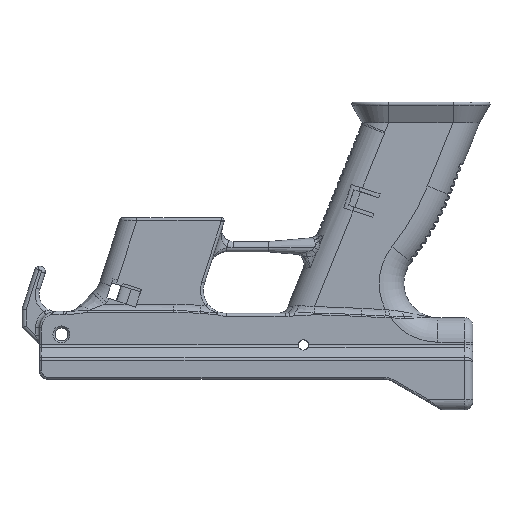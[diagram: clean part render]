
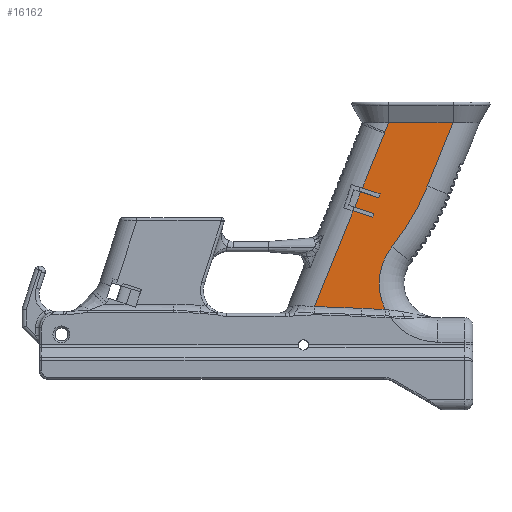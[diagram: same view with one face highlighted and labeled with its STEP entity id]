
A CAD part, front view. The second image highlights one B-rep face of the part: STEP entity #16162.
In plain terms, the highlighted planar face has unit normal (0, -1, 0).
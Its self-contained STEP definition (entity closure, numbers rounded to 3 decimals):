
#1591=FACE_OUTER_BOUND('',#2567,.T.);
#2567=EDGE_LOOP('',(#12655,#12656,#12657,#12658,#12659,#12660,#12661,#12662,
#12663,#12664,#12665,#12666,#12667,#12668,#12669,#12670,#12671));
#3439=CIRCLE('',#17698,696.304);
#3440=CIRCLE('',#17699,689.416);
#3441=CIRCLE('',#17700,28.63);
#3442=CIRCLE('',#17701,118.894);
#3443=CIRCLE('',#17702,17.);
#4932=LINE('',#29769,#5874);
#4947=LINE('',#29909,#5889);
#4948=LINE('',#29917,#5890);
#4990=LINE('',#31577,#5932);
#4991=LINE('',#31579,#5933);
#4992=LINE('',#31580,#5934);
#4993=LINE('',#31589,#5935);
#4994=LINE('',#31591,#5936);
#4995=LINE('',#31594,#5937);
#4996=LINE('',#31596,#5938);
#4997=LINE('',#31598,#5939);
#4998=LINE('',#31599,#5940);
#5874=VECTOR('',#20651,1000.);
#5889=VECTOR('',#20726,1000.);
#5890=VECTOR('',#20733,1000.);
#5932=VECTOR('',#20863,1000.);
#5933=VECTOR('',#20864,1000.);
#5934=VECTOR('',#20865,1000.);
#5935=VECTOR('',#20874,1000.);
#5936=VECTOR('',#20875,1000.);
#5937=VECTOR('',#20878,1000.);
#5938=VECTOR('',#20879,1000.);
#5939=VECTOR('',#20880,1000.);
#5940=VECTOR('',#20881,1000.);
#7390=VERTEX_POINT('',#29734);
#7392=VERTEX_POINT('',#29768);
#7418=VERTEX_POINT('',#29901);
#7419=VERTEX_POINT('',#29908);
#7422=VERTEX_POINT('',#29914);
#7423=VERTEX_POINT('',#29916);
#7505=VERTEX_POINT('',#31575);
#7506=VERTEX_POINT('',#31576);
#7507=VERTEX_POINT('',#31578);
#7508=VERTEX_POINT('',#31581);
#7509=VERTEX_POINT('',#31583);
#7510=VERTEX_POINT('',#31585);
#7511=VERTEX_POINT('',#31588);
#7512=VERTEX_POINT('',#31590);
#7513=VERTEX_POINT('',#31593);
#7514=VERTEX_POINT('',#31595);
#7515=VERTEX_POINT('',#31597);
#9336=EDGE_CURVE('',#7390,#7392,#4932,.T.);
#9378=EDGE_CURVE('',#7418,#7419,#4947,.T.);
#9382=EDGE_CURVE('',#7422,#7423,#4948,.T.);
#9511=EDGE_CURVE('',#7505,#7506,#4990,.T.);
#9512=EDGE_CURVE('',#7505,#7507,#4991,.T.);
#9513=EDGE_CURVE('',#7507,#7419,#4992,.T.);
#9514=EDGE_CURVE('',#7508,#7418,#3439,.T.);
#9515=EDGE_CURVE('',#7509,#7508,#3440,.T.);
#9516=EDGE_CURVE('',#7510,#7509,#3441,.T.);
#9517=EDGE_CURVE('',#7392,#7510,#3442,.T.);
#9518=EDGE_CURVE('',#7511,#7390,#4993,.T.);
#9519=EDGE_CURVE('',#7511,#7512,#4994,.T.);
#9520=EDGE_CURVE('',#7423,#7512,#3443,.T.);
#9521=EDGE_CURVE('',#7422,#7513,#4995,.T.);
#9522=EDGE_CURVE('',#7513,#7514,#4996,.T.);
#9523=EDGE_CURVE('',#7515,#7514,#4997,.T.);
#9524=EDGE_CURVE('',#7506,#7515,#4998,.T.);
#12655=ORIENTED_EDGE('',*,*,#9511,.F.);
#12656=ORIENTED_EDGE('',*,*,#9512,.T.);
#12657=ORIENTED_EDGE('',*,*,#9513,.T.);
#12658=ORIENTED_EDGE('',*,*,#9378,.F.);
#12659=ORIENTED_EDGE('',*,*,#9514,.F.);
#12660=ORIENTED_EDGE('',*,*,#9515,.F.);
#12661=ORIENTED_EDGE('',*,*,#9516,.F.);
#12662=ORIENTED_EDGE('',*,*,#9517,.F.);
#12663=ORIENTED_EDGE('',*,*,#9336,.F.);
#12664=ORIENTED_EDGE('',*,*,#9518,.F.);
#12665=ORIENTED_EDGE('',*,*,#9519,.T.);
#12666=ORIENTED_EDGE('',*,*,#9520,.F.);
#12667=ORIENTED_EDGE('',*,*,#9382,.F.);
#12668=ORIENTED_EDGE('',*,*,#9521,.T.);
#12669=ORIENTED_EDGE('',*,*,#9522,.T.);
#12670=ORIENTED_EDGE('',*,*,#9523,.F.);
#12671=ORIENTED_EDGE('',*,*,#9524,.F.);
#15610=PLANE('',#17697);
#16162=ADVANCED_FACE('',(#1591),#15610,.T.);
#17697=AXIS2_PLACEMENT_3D('',#31574,#20861,#20862);
#17698=AXIS2_PLACEMENT_3D('',#31582,#20866,#20867);
#17699=AXIS2_PLACEMENT_3D('',#31584,#20868,#20869);
#17700=AXIS2_PLACEMENT_3D('',#31586,#20870,#20871);
#17701=AXIS2_PLACEMENT_3D('',#31587,#20872,#20873);
#17702=AXIS2_PLACEMENT_3D('',#31592,#20876,#20877);
#20651=DIRECTION('',(-0.375,0.,-0.927));
#20726=DIRECTION('',(0.375,0.,0.927));
#20733=DIRECTION('',(0.375,0.,0.927));
#20861=DIRECTION('center_axis',(0.,-1.,0.));
#20862=DIRECTION('ref_axis',(0.,0.,-1.));
#20863=DIRECTION('',(-0.952,0.,0.305));
#20864=DIRECTION('',(-0.305,0.,-0.952));
#20865=DIRECTION('',(-0.952,0.,0.305));
#20866=DIRECTION('center_axis',(0.,-1.,0.));
#20867=DIRECTION('ref_axis',(-0.054,0.,-0.999));
#20868=DIRECTION('center_axis',(0.,1.,0.));
#20869=DIRECTION('ref_axis',(0.037,0.,0.999));
#20870=DIRECTION('center_axis',(0.,-1.,0.));
#20871=DIRECTION('ref_axis',(0.782,0.,-0.624));
#20872=DIRECTION('center_axis',(0.,1.,0.));
#20873=DIRECTION('ref_axis',(0.891,0.,-0.454));
#20874=DIRECTION('',(1.,0.,0.));
#20875=DIRECTION('',(-0.375,0.,-0.927));
#20876=DIRECTION('center_axis',(0.,-1.,0.));
#20877=DIRECTION('ref_axis',(0.992,0.,0.126));
#20878=DIRECTION('',(0.952,0.,-0.305));
#20879=DIRECTION('',(-0.305,0.,-0.952));
#20880=DIRECTION('',(0.952,0.,-0.305));
#20881=DIRECTION('',(0.375,0.,0.927));
#29734=CARTESIAN_POINT('',(121.365,-14.625,27.958));
#29768=CARTESIAN_POINT('',(108.893,-14.625,-2.912));
#29769=CARTESIAN_POINT('',(111.761,-14.625,4.188));
#29901=CARTESIAN_POINT('',(53.832,-14.625,-61.703));
#29908=CARTESIAN_POINT('',(72.662,-14.625,-15.097));
#29909=CARTESIAN_POINT('',(70.22,-14.625,-21.141));
#29914=CARTESIAN_POINT('',(77.169,-14.625,-3.94));
#29916=CARTESIAN_POINT('',(87.937,-14.625,22.71));
#29917=CARTESIAN_POINT('',(70.22,-14.625,-21.141));
#31574=CARTESIAN_POINT('Origin',(86.464,-14.625,-15.081));
#31575=CARTESIAN_POINT('',(82.782,-14.625,-16.238));
#31576=CARTESIAN_POINT('',(73.413,-14.625,-13.237));
#31577=CARTESIAN_POINT('',(2.985,-14.625,9.32));
#31578=CARTESIAN_POINT('',(82.172,-14.625,-18.143));
#31579=CARTESIAN_POINT('',(79.797,-14.625,-25.559));
#31580=CARTESIAN_POINT('',(2.375,-14.625,7.416));
#31581=CARTESIAN_POINT('',(76.954,-14.625,-62.561));
#31582=CARTESIAN_POINT('Origin',(39.557,-14.625,-757.86));
#31583=CARTESIAN_POINT('',(88.326,-14.625,-63.079));
#31584=CARTESIAN_POINT('Origin',(113.981,-14.625,625.86));
#31585=CARTESIAN_POINT('',(91.6,-14.625,-32.517));
#31586=CARTESIAN_POINT('Origin',(113.981,-14.625,-50.37));
#31587=CARTESIAN_POINT('Origin',(-1.344,-14.625,41.627));
#31588=CARTESIAN_POINT('',(90.04,-14.625,27.958));
#31589=CARTESIAN_POINT('',(69.665,-14.625,27.958));
#31590=CARTESIAN_POINT('',(88.199,-14.625,23.402));
#31591=CARTESIAN_POINT('',(106.929,-14.625,69.761));
#31592=CARTESIAN_POINT('Origin',(72.175,-14.625,29.078));
#31593=CARTESIAN_POINT('',(85.832,-14.625,-6.715));
#31594=CARTESIAN_POINT('',(88.836,-14.625,-7.677));
#31595=CARTESIAN_POINT('',(85.222,-14.625,-8.619));
#31596=CARTESIAN_POINT('',(79.797,-14.625,-25.559));
#31597=CARTESIAN_POINT('',(76.418,-14.625,-5.799));
#31598=CARTESIAN_POINT('',(88.226,-14.625,-9.581));
#31599=CARTESIAN_POINT('',(70.22,-14.625,-21.141));
